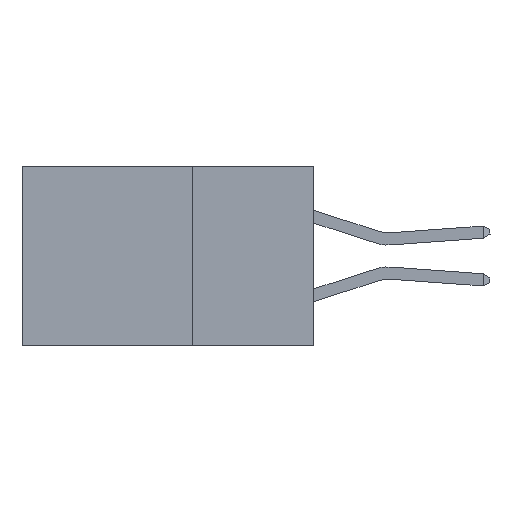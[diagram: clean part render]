
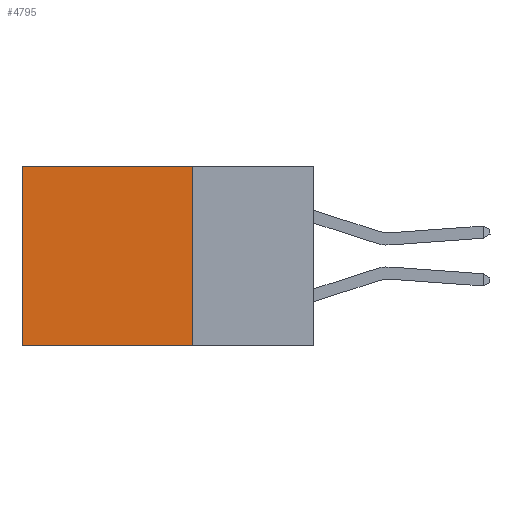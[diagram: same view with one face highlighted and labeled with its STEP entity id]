
A CAD part, left-side view. The second image highlights one B-rep face of the part: STEP entity #4795.
In plain terms, the highlighted planar face has unit normal (-1, 0, 0).
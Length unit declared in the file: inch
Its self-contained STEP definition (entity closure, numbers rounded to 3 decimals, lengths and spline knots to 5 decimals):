
#826 = DIRECTION ( 'NONE',  ( 0., 0., -1. ) ) ;
#1094 = EDGE_CURVE ( 'NONE', #13892, #19050, #8648, .T. ) ;
#1118 = EDGE_CURVE ( 'NONE', #14756, #11057, #3610, .T. ) ;
#1219 = CARTESIAN_POINT ( 'NONE',  ( 0.2875, 0.6, 0. ) ) ;
#2525 = VECTOR ( 'NONE', #5230, 39.37008 ) ;
#2796 = ORIENTED_EDGE ( 'NONE', *, *, #19272, .F. ) ;
#3470 = CARTESIAN_POINT ( 'NONE',  ( 0.2875, 0.25, -0.37 ) ) ;
#3610 = LINE ( 'NONE', #11760, #5605 ) ;
#4795 = ADVANCED_FACE ( 'NONE', ( #19985 ), #16686, .F. ) ;
#5230 = DIRECTION ( 'NONE',  ( 0., 1., 0. ) ) ;
#5352 = CARTESIAN_POINT ( 'NONE',  ( 0.2875, 0.25, 0. ) ) ;
#5558 = DIRECTION ( 'NONE',  ( 1., 0., 0. ) ) ;
#5605 = VECTOR ( 'NONE', #16675, 39.37008 ) ;
#7281 = EDGE_CURVE ( 'NONE', #11057, #19050, #9288, .T. ) ;
#7302 = EDGE_LOOP ( 'NONE', ( #10057, #9792, #2796, #17514 ) ) ;
#7507 = CARTESIAN_POINT ( 'NONE',  ( 0.2875, 0.6, -0.37 ) ) ;
#7883 = CARTESIAN_POINT ( 'NONE',  ( 0.2875, 0.6, 0. ) ) ;
#8105 = AXIS2_PLACEMENT_3D ( 'NONE', #5352, #5558, #15192 ) ;
#8648 = LINE ( 'NONE', #19858, #2525 ) ;
#9288 = LINE ( 'NONE', #7883, #10747 ) ;
#9792 = ORIENTED_EDGE ( 'NONE', *, *, #1094, .F. ) ;
#10057 = ORIENTED_EDGE ( 'NONE', *, *, #7281, .T. ) ;
#10747 = VECTOR ( 'NONE', #14197, 39.37008 ) ;
#11057 = VERTEX_POINT ( 'NONE', #1219 ) ;
#11760 = CARTESIAN_POINT ( 'NONE',  ( 0.2875, 0.25, 0. ) ) ;
#12178 = LINE ( 'NONE', #13879, #17180 ) ;
#13243 = CARTESIAN_POINT ( 'NONE',  ( 0.2875, 0.25, 0. ) ) ;
#13879 = CARTESIAN_POINT ( 'NONE',  ( 0.2875, 0.25, 0. ) ) ;
#13892 = VERTEX_POINT ( 'NONE', #3470 ) ;
#14197 = DIRECTION ( 'NONE',  ( 0., 0., -1. ) ) ;
#14756 = VERTEX_POINT ( 'NONE', #13243 ) ;
#15192 = DIRECTION ( 'NONE',  ( 0., 0., -1. ) ) ;
#16675 = DIRECTION ( 'NONE',  ( 0., 1., 0. ) ) ;
#16686 = PLANE ( 'NONE',  #8105 ) ;
#17180 = VECTOR ( 'NONE', #826, 39.37008 ) ;
#17514 = ORIENTED_EDGE ( 'NONE', *, *, #1118, .T. ) ;
#19050 = VERTEX_POINT ( 'NONE', #7507 ) ;
#19272 = EDGE_CURVE ( 'NONE', #14756, #13892, #12178, .T. ) ;
#19858 = CARTESIAN_POINT ( 'NONE',  ( 0.2875, 0.25, -0.37 ) ) ;
#19985 = FACE_OUTER_BOUND ( 'NONE', #7302, .T. ) ;
